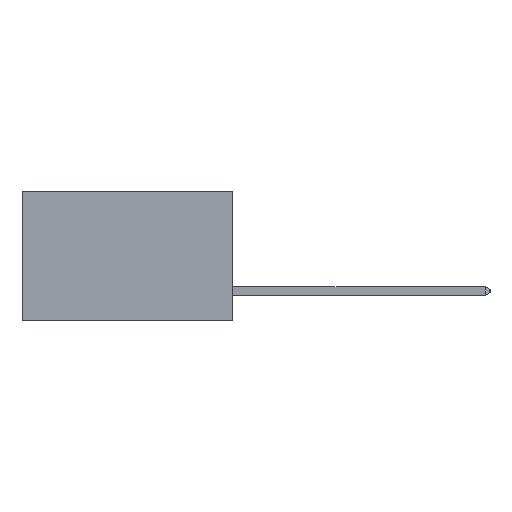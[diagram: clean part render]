
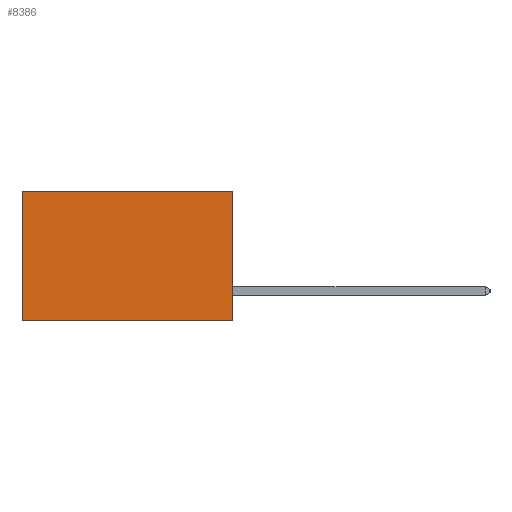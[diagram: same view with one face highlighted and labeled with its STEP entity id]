
A CAD part, left-side view. The second image highlights one B-rep face of the part: STEP entity #8386.
In plain terms, the highlighted planar face has unit normal (-1, 0, 0).
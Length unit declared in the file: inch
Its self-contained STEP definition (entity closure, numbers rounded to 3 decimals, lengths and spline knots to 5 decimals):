
#585 = VECTOR ( 'NONE', #1693, 39.37008 ) ;
#1693 = DIRECTION ( 'NONE',  ( 0., 1., 0. ) ) ;
#2345 = EDGE_CURVE ( 'NONE', #7293, #2519, #6907, .T. ) ;
#2519 = VERTEX_POINT ( 'NONE', #23324 ) ;
#3469 = CARTESIAN_POINT ( 'NONE',  ( 0.2875, 0., -0.37 ) ) ;
#3516 = DIRECTION ( 'NONE',  ( 0., 0., -1. ) ) ;
#3623 = PLANE ( 'NONE',  #13796 ) ;
#6907 = LINE ( 'NONE', #14682, #585 ) ;
#7293 = VERTEX_POINT ( 'NONE', #16232 ) ;
#7713 = EDGE_CURVE ( 'NONE', #7293, #14134, #24001, .T. ) ;
#7912 = DIRECTION ( 'NONE',  ( 1., 0., 0. ) ) ;
#8248 = VERTEX_POINT ( 'NONE', #26022 ) ;
#8386 = ADVANCED_FACE ( 'NONE', ( #22307 ), #3623, .F. ) ;
#9419 = DIRECTION ( 'NONE',  ( 0., 0., -1. ) ) ;
#9431 = ORIENTED_EDGE ( 'NONE', *, *, #2345, .T. ) ;
#10121 = VECTOR ( 'NONE', #3516, 39.37008 ) ;
#11396 = ORIENTED_EDGE ( 'NONE', *, *, #7713, .F. ) ;
#11812 = VECTOR ( 'NONE', #12291, 39.37008 ) ;
#12291 = DIRECTION ( 'NONE',  ( 0., 1., 0. ) ) ;
#13796 = AXIS2_PLACEMENT_3D ( 'NONE', #20553, #7912, #22697 ) ;
#14134 = VERTEX_POINT ( 'NONE', #3469 ) ;
#14682 = CARTESIAN_POINT ( 'NONE',  ( 0.2875, 0., 0. ) ) ;
#14884 = EDGE_CURVE ( 'NONE', #14134, #8248, #22374, .T. ) ;
#15535 = EDGE_CURVE ( 'NONE', #2519, #8248, #26976, .T. ) ;
#16232 = CARTESIAN_POINT ( 'NONE',  ( 0.2875, 0., 0. ) ) ;
#17707 = VECTOR ( 'NONE', #9419, 39.37008 ) ;
#17819 = CARTESIAN_POINT ( 'NONE',  ( 0.2875, 0., 0. ) ) ;
#18339 = CARTESIAN_POINT ( 'NONE',  ( 0.2875, 0.6, 0. ) ) ;
#19824 = ORIENTED_EDGE ( 'NONE', *, *, #15535, .T. ) ;
#20520 = EDGE_LOOP ( 'NONE', ( #19824, #26959, #11396, #9431 ) ) ;
#20553 = CARTESIAN_POINT ( 'NONE',  ( 0.2875, 0., 0. ) ) ;
#22307 = FACE_OUTER_BOUND ( 'NONE', #20520, .T. ) ;
#22374 = LINE ( 'NONE', #27063, #11812 ) ;
#22697 = DIRECTION ( 'NONE',  ( 0., 0., -1. ) ) ;
#23324 = CARTESIAN_POINT ( 'NONE',  ( 0.2875, 0.6, 0. ) ) ;
#24001 = LINE ( 'NONE', #17819, #17707 ) ;
#26022 = CARTESIAN_POINT ( 'NONE',  ( 0.2875, 0.6, -0.37 ) ) ;
#26959 = ORIENTED_EDGE ( 'NONE', *, *, #14884, .F. ) ;
#26976 = LINE ( 'NONE', #18339, #10121 ) ;
#27063 = CARTESIAN_POINT ( 'NONE',  ( 0.2875, 0., -0.37 ) ) ;
